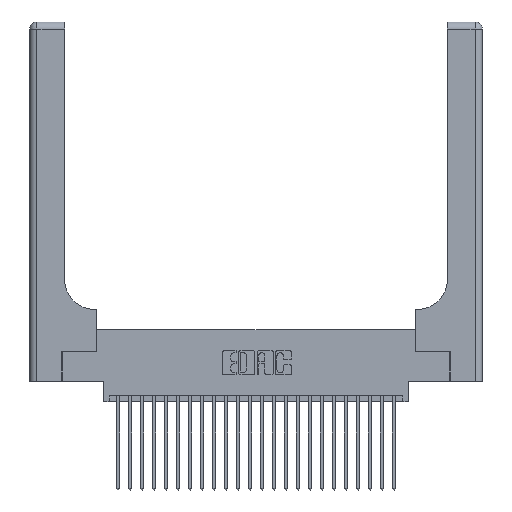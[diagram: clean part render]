
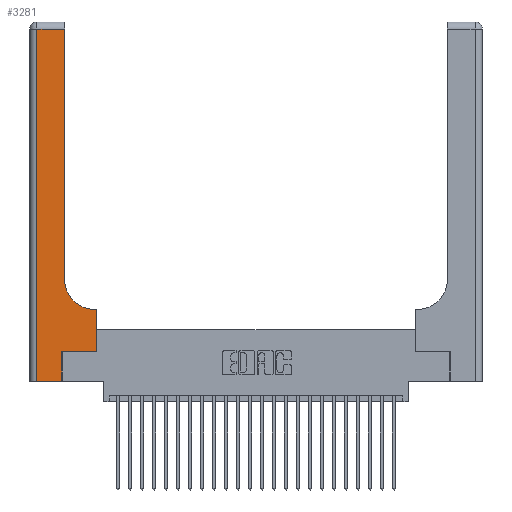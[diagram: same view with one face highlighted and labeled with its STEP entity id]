
A CAD part, top view. The second image highlights one B-rep face of the part: STEP entity #3281.
In plain terms, the highlighted planar face has unit normal (0, 0, 1).
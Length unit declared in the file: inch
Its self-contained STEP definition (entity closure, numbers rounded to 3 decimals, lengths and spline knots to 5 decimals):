
#15 = ORIENTED_EDGE ( 'NONE', *, *, #105, .T. ) ;
#105 = EDGE_CURVE ( 'NONE', #863, #8581, #25619, .T. ) ;
#563 = DIRECTION ( 'NONE',  ( 0., 1., 0. ) ) ;
#660 = ORIENTED_EDGE ( 'NONE', *, *, #3795, .T. ) ;
#813 = VECTOR ( 'NONE', #17412, 39.37008 ) ;
#838 = FACE_OUTER_BOUND ( 'NONE', #23014, .T. ) ;
#850 = CARTESIAN_POINT ( 'NONE',  ( 0., 0., 0.37 ) ) ;
#863 = VERTEX_POINT ( 'NONE', #5439 ) ;
#1092 = CARTESIAN_POINT ( 'NONE',  ( 0.2915, 0.6, 0.37 ) ) ;
#2192 = CARTESIAN_POINT ( 'NONE',  ( 0.06, 3., 0.37 ) ) ;
#2580 = CARTESIAN_POINT ( 'NONE',  ( 0.269, 0., 0.37 ) ) ;
#2587 = VERTEX_POINT ( 'NONE', #17310 ) ;
#3036 = CARTESIAN_POINT ( 'NONE',  ( 0.269, 0.25, 0.37 ) ) ;
#3252 = DIRECTION ( 'NONE',  ( 0., -1., 0. ) ) ;
#3281 = ADVANCED_FACE ( 'NONE', ( #838 ), #13676, .F. ) ;
#3603 = CARTESIAN_POINT ( 'NONE',  ( 0.2915, 3., 0.37 ) ) ;
#3795 = EDGE_CURVE ( 'NONE', #8581, #20634, #17338, .T. ) ;
#3875 = VECTOR ( 'NONE', #3252, 39.37008 ) ;
#5181 = VECTOR ( 'NONE', #17481, 39.37008 ) ;
#5439 = CARTESIAN_POINT ( 'NONE',  ( 0.06, 2.94, 0.37 ) ) ;
#5455 = VERTEX_POINT ( 'NONE', #15522 ) ;
#5464 = DIRECTION ( 'NONE',  ( -1., 0., 0. ) ) ;
#5846 = CIRCLE ( 'NONE', #16689, 0.25 ) ;
#5878 = VECTOR ( 'NONE', #20786, 39.37008 ) ;
#6180 = VECTOR ( 'NONE', #563, 39.37008 ) ;
#6491 = CARTESIAN_POINT ( 'NONE',  ( 0., 2.94, 0.37 ) ) ;
#7447 = CARTESIAN_POINT ( 'NONE',  ( 0.2915, 0.85, 0.37 ) ) ;
#7506 = EDGE_CURVE ( 'NONE', #19405, #18305, #13118, .T. ) ;
#7627 = VECTOR ( 'NONE', #14705, 39.37008 ) ;
#8122 = ORIENTED_EDGE ( 'NONE', *, *, #17792, .T. ) ;
#8504 = CARTESIAN_POINT ( 'NONE',  ( 0.5585, 0.25, 0.37 ) ) ;
#8581 = VERTEX_POINT ( 'NONE', #23247 ) ;
#9404 = CARTESIAN_POINT ( 'NONE',  ( 0.5415, 0.85, 0.37 ) ) ;
#9542 = CARTESIAN_POINT ( 'NONE',  ( 0., 3., 0.37 ) ) ;
#11012 = LINE ( 'NONE', #2580, #6180 ) ;
#11091 = EDGE_CURVE ( 'NONE', #17194, #2587, #25042, .T. ) ;
#11473 = DIRECTION ( 'NONE',  ( 1., 0., 0. ) ) ;
#11478 = EDGE_CURVE ( 'NONE', #5455, #17194, #5846, .T. ) ;
#13118 = LINE ( 'NONE', #8504, #7627 ) ;
#13639 = LINE ( 'NONE', #1092, #24433 ) ;
#13676 = PLANE ( 'NONE',  #21111 ) ;
#13910 = CARTESIAN_POINT ( 'NONE',  ( 0.5585, 0.25, 0.37 ) ) ;
#14638 = ORIENTED_EDGE ( 'NONE', *, *, #11478, .T. ) ;
#14705 = DIRECTION ( 'NONE',  ( 0., 1., 0. ) ) ;
#15522 = CARTESIAN_POINT ( 'NONE',  ( 0.5415, 0.6, 0.37 ) ) ;
#15524 = VECTOR ( 'NONE', #18017, 39.37008 ) ;
#15580 = DIRECTION ( 'NONE',  ( -1., 0., 0. ) ) ;
#15808 = VERTEX_POINT ( 'NONE', #16183 ) ;
#16169 = LINE ( 'NONE', #6491, #5878 ) ;
#16183 = CARTESIAN_POINT ( 'NONE',  ( 0.269, 0.25, 0.37 ) ) ;
#16689 = AXIS2_PLACEMENT_3D ( 'NONE', #9404, #23641, #11473 ) ;
#17194 = VERTEX_POINT ( 'NONE', #7447 ) ;
#17310 = CARTESIAN_POINT ( 'NONE',  ( 0.2915, 2.94, 0.37 ) ) ;
#17338 = LINE ( 'NONE', #850, #813 ) ;
#17412 = DIRECTION ( 'NONE',  ( 1., 0., 0. ) ) ;
#17481 = DIRECTION ( 'NONE',  ( 1., 0., 0. ) ) ;
#17777 = DIRECTION ( 'NONE',  ( 0., 0., -1. ) ) ;
#17792 = EDGE_CURVE ( 'NONE', #18305, #5455, #13639, .T. ) ;
#18017 = DIRECTION ( 'NONE',  ( 0., 1., 0. ) ) ;
#18153 = EDGE_CURVE ( 'NONE', #2587, #863, #16169, .T. ) ;
#18305 = VERTEX_POINT ( 'NONE', #21133 ) ;
#18880 = ORIENTED_EDGE ( 'NONE', *, *, #25434, .T. ) ;
#19405 = VERTEX_POINT ( 'NONE', #13910 ) ;
#20634 = VERTEX_POINT ( 'NONE', #25895 ) ;
#20786 = DIRECTION ( 'NONE',  ( -1., 0., 0. ) ) ;
#20872 = LINE ( 'NONE', #3036, #5181 ) ;
#21111 = AXIS2_PLACEMENT_3D ( 'NONE', #9542, #17777, #5464 ) ;
#21126 = ORIENTED_EDGE ( 'NONE', *, *, #11091, .T. ) ;
#21133 = CARTESIAN_POINT ( 'NONE',  ( 0.5585, 0.6, 0.37 ) ) ;
#22357 = ORIENTED_EDGE ( 'NONE', *, *, #7506, .T. ) ;
#23014 = EDGE_LOOP ( 'NONE', ( #21126, #25750, #15, #660, #18880, #26581, #22357, #8122, #14638 ) ) ;
#23247 = CARTESIAN_POINT ( 'NONE',  ( 0.06, 0., 0.37 ) ) ;
#23641 = DIRECTION ( 'NONE',  ( 0., 0., -1. ) ) ;
#24433 = VECTOR ( 'NONE', #15580, 39.37008 ) ;
#25042 = LINE ( 'NONE', #3603, #15524 ) ;
#25434 = EDGE_CURVE ( 'NONE', #20634, #15808, #11012, .T. ) ;
#25545 = EDGE_CURVE ( 'NONE', #15808, #19405, #20872, .T. ) ;
#25619 = LINE ( 'NONE', #2192, #3875 ) ;
#25750 = ORIENTED_EDGE ( 'NONE', *, *, #18153, .T. ) ;
#25895 = CARTESIAN_POINT ( 'NONE',  ( 0.269, 0., 0.37 ) ) ;
#26581 = ORIENTED_EDGE ( 'NONE', *, *, #25545, .T. ) ;
